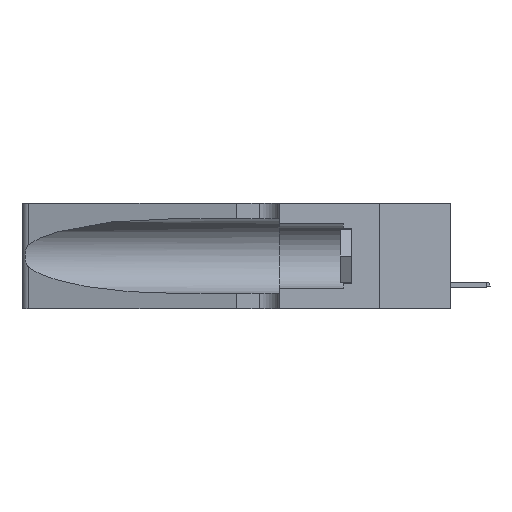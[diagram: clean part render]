
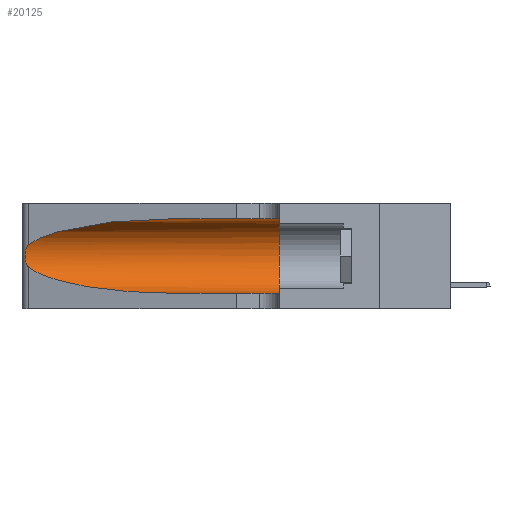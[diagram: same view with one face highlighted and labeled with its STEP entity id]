
A CAD part, left-side view. The second image highlights one B-rep face of the part: STEP entity #20125.
In plain terms, the highlighted cylindrical face has radius 3.308 mm (diameter 6.617 mm), a partial arc.
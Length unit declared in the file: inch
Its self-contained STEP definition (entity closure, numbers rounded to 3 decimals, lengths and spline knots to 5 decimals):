
#979 = FACE_OUTER_BOUND ( 'NONE', #4228, .T. ) ;
#1185 = ORIENTED_EDGE ( 'NONE', *, *, #6045, .T. ) ;
#1385 = VERTEX_POINT ( 'NONE', #10305 ) ;
#1584 = EDGE_CURVE ( 'NONE', #10696, #10094, #16099, .T. ) ;
#1716 = AXIS2_PLACEMENT_3D ( 'NONE', #22265, #20836, #9107 ) ;
#2204 = CARTESIAN_POINT ( 'NONE',  ( 0.25854, 1.2359, 0.20912 ) ) ;
#2333 = CARTESIAN_POINT ( 'NONE',  ( 0.26017, 1.23833, 0.17102 ) ) ;
#3000 = ORIENTED_EDGE ( 'NONE', *, *, #5527, .T. ) ;
#3950 = VERTEX_POINT ( 'NONE', #10370 ) ;
#4077 = CARTESIAN_POINT ( 'NONE',  ( 0.1305, 0.72297, 0.31525 ) ) ;
#4228 = EDGE_LOOP ( 'NONE', ( #1185, #3000, #22307, #13396, #6909, #6984 ) ) ;
#5527 = EDGE_CURVE ( 'NONE', #15928, #1385, #24709, .T. ) ;
#6045 = EDGE_CURVE ( 'NONE', #3950, #15928, #22441, .T. ) ;
#6150 = EDGE_CURVE ( 'NONE', #6238, #10094, #16765, .T. ) ;
#6238 = VERTEX_POINT ( 'NONE', #11318 ) ;
#6340 = CARTESIAN_POINT ( 'NONE',  ( 0.1305, 0.35, 0.31525 ) ) ;
#6909 = ORIENTED_EDGE ( 'NONE', *, *, #1584, .F. ) ;
#6984 = ORIENTED_EDGE ( 'NONE', *, *, #22986, .F. ) ;
#7044 = VECTOR ( 'NONE', #14711, 39.37008 ) ;
#8772 = CARTESIAN_POINT ( 'NONE',  ( 0.1305, 0.35, 0.185 ) ) ;
#9107 = DIRECTION ( 'NONE',  ( 0., 0., -1. ) ) ;
#9971 = CARTESIAN_POINT ( 'NONE',  ( 0.26075, 1.23896, 0.19203 ) ) ;
#10094 = VERTEX_POINT ( 'NONE', #21977 ) ;
#10305 = CARTESIAN_POINT ( 'NONE',  ( 0.25487, 1.22718, 0.14631 ) ) ;
#10370 = CARTESIAN_POINT ( 'NONE',  ( 0.1305, 0.72297, 0.31525 ) ) ;
#10696 = VERTEX_POINT ( 'NONE', #6340 ) ;
#11010 = CARTESIAN_POINT ( 'NONE',  ( 0.2373, 1.15595, 0.08982 ) ) ;
#11318 = CARTESIAN_POINT ( 'NONE',  ( 0.1305, 0.72297, 0.05475 ) ) ;
#11516 = CARTESIAN_POINT ( 'NONE',  ( 0.25787, 1.23484, 0.2124 ) ) ;
#12135 = CARTESIAN_POINT ( 'NONE',  ( 0.25639, 1.23186, 0.15144 ) ) ;
#12268 = CARTESIAN_POINT ( 'NONE',  ( 0.26075, 1.23896, 0.178 ) ) ;
#12878 = CARTESIAN_POINT ( 'NONE',  ( 0.25487, 1.22718, 0.22369 ) ) ;
#12945 = CARTESIAN_POINT ( 'NONE',  ( 0.18966, 0.96281, 0.05475 ) ) ;
#13396 = ORIENTED_EDGE ( 'NONE', *, *, #6150, .T. ) ;
#13879 = CARTESIAN_POINT ( 'NONE',  ( 0.2373, 1.15595, 0.28018 ) ) ;
#14005 = CARTESIAN_POINT ( 'NONE',  ( 0.18966, 0.96281, 0.31525 ) ) ;
#14376 = DIRECTION ( 'NONE',  ( 0., -1., 0. ) ) ;
#14621 = DIRECTION ( 'NONE',  ( 0., 1., 0. ) ) ;
#14711 = DIRECTION ( 'NONE',  ( 0., -1., 0. ) ) ;
#15318 = CARTESIAN_POINT ( 'NONE',  ( 0.25555, 1.22994, 0.2215 ) ) ;
#15928 = VERTEX_POINT ( 'NONE', #12878 ) ;
#15946 = CARTESIAN_POINT ( 'NONE',  ( 0.25555, 1.22993, 0.14849 ) ) ;
#16099 = CIRCLE ( 'NONE', #23865, 0.13025 ) ;
#16478 = CYLINDRICAL_SURFACE ( 'NONE', #1716, 0.13025 ) ;
#16765 = LINE ( 'NONE', #24240, #22235 ) ;
#17097 = CARTESIAN_POINT ( 'NONE',  ( 0.1305, 0.72297, 0.05475 ) ) ;
#18093 = CARTESIAN_POINT ( 'NONE',  ( 0.25789, 1.23486, 0.15765 ) ) ;
#18131 = EDGE_CURVE ( 'NONE', #1385, #6238, #25056, .T. ) ;
#18158 = CARTESIAN_POINT ( 'NONE',  ( 0.1305, 1.61858, 0.31525 ) ) ;
#19612 = CARTESIAN_POINT ( 'NONE',  ( 0.25487, 1.22718, 0.22369 ) ) ;
#20125 = ADVANCED_FACE ( 'NONE', ( #979 ), #16478, .F. ) ;
#20836 = DIRECTION ( 'NONE',  ( 0., -1., 0. ) ) ;
#20970 = CARTESIAN_POINT ( 'NONE',  ( 0.25487, 1.22718, 0.14631 ) ) ;
#21208 = CARTESIAN_POINT ( 'NONE',  ( 0.25639, 1.23184, 0.21858 ) ) ;
#21966 = CARTESIAN_POINT ( 'NONE',  ( 0.26018, 1.23835, 0.19895 ) ) ;
#21977 = CARTESIAN_POINT ( 'NONE',  ( 0.1305, 0.35, 0.05475 ) ) ;
#22235 = VECTOR ( 'NONE', #14376, 39.37008 ) ;
#22265 = CARTESIAN_POINT ( 'NONE',  ( 0.1305, 1.61858, 0.185 ) ) ;
#22307 = ORIENTED_EDGE ( 'NONE', *, *, #18131, .T. ) ;
#22425 = DIRECTION ( 'NONE',  ( 0., 0., 1. ) ) ;
#22441 =( BOUNDED_CURVE ( )  B_SPLINE_CURVE ( 3, ( #4077, #14005, #13879, #19612 ),
 .UNSPECIFIED., .F., .F. ) 
 B_SPLINE_CURVE_WITH_KNOTS ( ( 4, 4 ),
 ( 1.5708, 2.84003 ),
 .UNSPECIFIED. ) 
 CURVE ( )  GEOMETRIC_REPRESENTATION_ITEM ( )  RATIONAL_B_SPLINE_CURVE ( ( 1., 0.87, 0.87, 1. ) ) 
 REPRESENTATION_ITEM ( '' )  );
#22986 = EDGE_CURVE ( 'NONE', #3950, #10696, #23952, .T. ) ;
#23635 = CARTESIAN_POINT ( 'NONE',  ( 0.25487, 1.22718, 0.14631 ) ) ;
#23768 = CARTESIAN_POINT ( 'NONE',  ( 0.25856, 1.23593, 0.16098 ) ) ;
#23865 = AXIS2_PLACEMENT_3D ( 'NONE', #8772, #14621, #22425 ) ;
#23952 = LINE ( 'NONE', #18158, #7044 ) ;
#24240 = CARTESIAN_POINT ( 'NONE',  ( 0.1305, 1.61858, 0.05475 ) ) ;
#24709 = B_SPLINE_CURVE_WITH_KNOTS ( 'NONE', 3,
 ( #25052, #15318, #21208, #11516, #2204, #21966, #9971, #12268, #2333, #23768, #18093, #12135, #15946, #23635 ),
 .UNSPECIFIED., .F., .F.,
 ( 4, 2, 2, 2, 2, 2, 4 ),
 ( 0., 0.00027, 0.00053, 0.00107, 0.0016, 0.00187, 0.00214 ),
 .UNSPECIFIED. ) ;
#25052 = CARTESIAN_POINT ( 'NONE',  ( 0.25487, 1.22718, 0.22369 ) ) ;
#25056 =( BOUNDED_CURVE ( )  B_SPLINE_CURVE ( 3, ( #20970, #11010, #12945, #17097 ),
 .UNSPECIFIED., .F., .F. ) 
 B_SPLINE_CURVE_WITH_KNOTS ( ( 4, 4 ),
 ( 3.44316, 4.71239 ),
 .UNSPECIFIED. ) 
 CURVE ( )  GEOMETRIC_REPRESENTATION_ITEM ( )  RATIONAL_B_SPLINE_CURVE ( ( 1., 0.87, 0.87, 1. ) ) 
 REPRESENTATION_ITEM ( '' )  );
